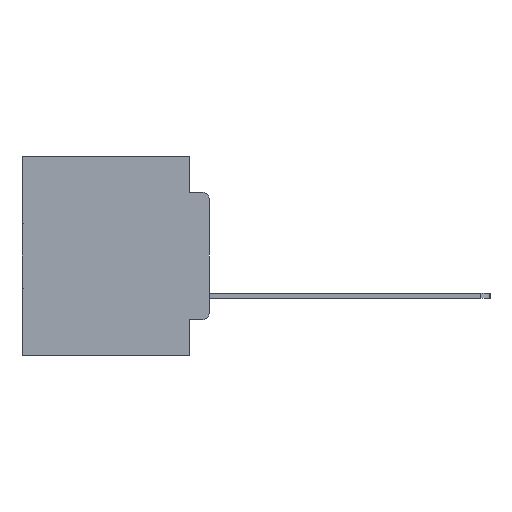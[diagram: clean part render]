
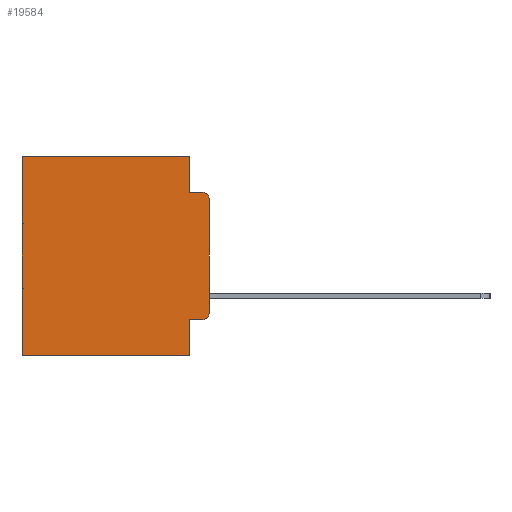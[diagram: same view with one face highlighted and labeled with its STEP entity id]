
A CAD part, left-side view. The second image highlights one B-rep face of the part: STEP entity #19584.
In plain terms, the highlighted planar face has unit normal (-1, 0, 0).
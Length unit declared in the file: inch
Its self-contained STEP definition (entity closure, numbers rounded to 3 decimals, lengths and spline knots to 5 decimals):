
#399 = CARTESIAN_POINT ( 'NONE',  ( 0.298, 0.473, -0.5 ) ) ;
#1230 = VERTEX_POINT ( 'NONE', #14262 ) ;
#1548 = CARTESIAN_POINT ( 'NONE',  ( 0.298, 0., -0.5 ) ) ;
#1728 = DIRECTION ( 'NONE',  ( 0., -1., 0. ) ) ;
#1893 = EDGE_CURVE ( 'NONE', #27802, #9238, #28339, .T. ) ;
#2396 = LINE ( 'NONE', #1548, #15229 ) ;
#2546 = CARTESIAN_POINT ( 'NONE',  ( 0.298, 0.02, -0.4115 ) ) ;
#2710 = CARTESIAN_POINT ( 'NONE',  ( 0.298, 0.051, -0.5 ) ) ;
#2961 = CARTESIAN_POINT ( 'NONE',  ( 0.298, 0.051, -0.0885 ) ) ;
#3117 = DIRECTION ( 'NONE',  ( 1., 0., 0. ) ) ;
#3260 = EDGE_LOOP ( 'NONE', ( #10660, #15494, #16611, #5345, #18315, #19833, #30527, #13112, #24665, #4795 ) ) ;
#3614 = DIRECTION ( 'NONE',  ( -1., 0., 0. ) ) ;
#4443 = CARTESIAN_POINT ( 'NONE',  ( 0.298, 0., 0. ) ) ;
#4523 = VERTEX_POINT ( 'NONE', #399 ) ;
#4795 = ORIENTED_EDGE ( 'NONE', *, *, #14055, .T. ) ;
#5158 = EDGE_CURVE ( 'NONE', #26946, #17206, #25175, .T. ) ;
#5345 = ORIENTED_EDGE ( 'NONE', *, *, #13250, .F. ) ;
#5708 = AXIS2_PLACEMENT_3D ( 'NONE', #12747, #29348, #15118 ) ;
#6300 = VERTEX_POINT ( 'NONE', #28837 ) ;
#6594 = VECTOR ( 'NONE', #21126, 39.37008 ) ;
#6880 = CARTESIAN_POINT ( 'NONE',  ( 0.298, 0.473, 0. ) ) ;
#7714 = DIRECTION ( 'NONE',  ( 0., 1., 0. ) ) ;
#8051 = VERTEX_POINT ( 'NONE', #2710 ) ;
#9105 = CARTESIAN_POINT ( 'NONE',  ( 0.298, 0.051, 0. ) ) ;
#9238 = VERTEX_POINT ( 'NONE', #14763 ) ;
#9301 = DIRECTION ( 'NONE',  ( 0., 0., -1. ) ) ;
#9405 = AXIS2_PLACEMENT_3D ( 'NONE', #18001, #3614, #20428 ) ;
#10660 = ORIENTED_EDGE ( 'NONE', *, *, #1893, .F. ) ;
#10932 = AXIS2_PLACEMENT_3D ( 'NONE', #17502, #3117, #19942 ) ;
#11236 = VECTOR ( 'NONE', #21817, 39.37008 ) ;
#12475 = CIRCLE ( 'NONE', #9405, 0.02 ) ;
#12482 = LINE ( 'NONE', #29075, #24395 ) ;
#12747 = CARTESIAN_POINT ( 'NONE',  ( 0.298, 0.02, -0.3915 ) ) ;
#13112 = ORIENTED_EDGE ( 'NONE', *, *, #17889, .F. ) ;
#13146 = EDGE_CURVE ( 'NONE', #8051, #4523, #2396, .T. ) ;
#13250 = EDGE_CURVE ( 'NONE', #25063, #26946, #18600, .T. ) ;
#13692 = CIRCLE ( 'NONE', #5708, 0.02 ) ;
#14055 = EDGE_CURVE ( 'NONE', #22486, #9238, #13692, .T. ) ;
#14067 = VECTOR ( 'NONE', #9301, 39.37008 ) ;
#14262 = CARTESIAN_POINT ( 'NONE',  ( 0.298, 0.473, 0. ) ) ;
#14763 = CARTESIAN_POINT ( 'NONE',  ( 0.298, 0., -0.3915 ) ) ;
#15104 = PLANE ( 'NONE',  #10932 ) ;
#15118 = DIRECTION ( 'NONE',  ( 0., 0., -1. ) ) ;
#15187 = VECTOR ( 'NONE', #1728, 39.37008 ) ;
#15229 = VECTOR ( 'NONE', #18423, 39.37008 ) ;
#15494 = ORIENTED_EDGE ( 'NONE', *, *, #28383, .T. ) ;
#15580 = EDGE_CURVE ( 'NONE', #25063, #1230, #12482, .T. ) ;
#15688 = VECTOR ( 'NONE', #21330, 39.37008 ) ;
#16611 = ORIENTED_EDGE ( 'NONE', *, *, #5158, .F. ) ;
#17206 = VERTEX_POINT ( 'NONE', #23819 ) ;
#17361 = DIRECTION ( 'NONE',  ( 0., -1., 0. ) ) ;
#17502 = CARTESIAN_POINT ( 'NONE',  ( 0.298, 0., 0. ) ) ;
#17818 = CARTESIAN_POINT ( 'NONE',  ( 0.298, 0., -0.1085 ) ) ;
#17889 = EDGE_CURVE ( 'NONE', #6300, #8051, #22432, .T. ) ;
#18001 = CARTESIAN_POINT ( 'NONE',  ( 0.298, 0.02, -0.1085 ) ) ;
#18114 = VECTOR ( 'NONE', #17361, 39.37008 ) ;
#18204 = LINE ( 'NONE', #25669, #15187 ) ;
#18315 = ORIENTED_EDGE ( 'NONE', *, *, #15580, .T. ) ;
#18423 = DIRECTION ( 'NONE',  ( 0., 1., 0. ) ) ;
#18600 = LINE ( 'NONE', #25910, #6594 ) ;
#19226 = CARTESIAN_POINT ( 'NONE',  ( 0.298, 0.051, 0. ) ) ;
#19584 = ADVANCED_FACE ( 'NONE', ( #26059 ), #15104, .F. ) ;
#19833 = ORIENTED_EDGE ( 'NONE', *, *, #20341, .T. ) ;
#19942 = DIRECTION ( 'NONE',  ( 0., 0., -1. ) ) ;
#20341 = EDGE_CURVE ( 'NONE', #1230, #4523, #22661, .T. ) ;
#20428 = DIRECTION ( 'NONE',  ( 0., 0., -1. ) ) ;
#21126 = DIRECTION ( 'NONE',  ( 0., 0., -1. ) ) ;
#21330 = DIRECTION ( 'NONE',  ( 0., 0., -1. ) ) ;
#21522 = CARTESIAN_POINT ( 'NONE',  ( 0.298, 0.051, -0.0885 ) ) ;
#21817 = DIRECTION ( 'NONE',  ( 0., 0., -1. ) ) ;
#22432 = LINE ( 'NONE', #19226, #11236 ) ;
#22486 = VERTEX_POINT ( 'NONE', #2546 ) ;
#22661 = LINE ( 'NONE', #6880, #14067 ) ;
#23819 = CARTESIAN_POINT ( 'NONE',  ( 0.298, 0.02, -0.0885 ) ) ;
#24395 = VECTOR ( 'NONE', #7714, 39.37008 ) ;
#24665 = ORIENTED_EDGE ( 'NONE', *, *, #25683, .T. ) ;
#25063 = VERTEX_POINT ( 'NONE', #9105 ) ;
#25175 = LINE ( 'NONE', #2961, #18114 ) ;
#25669 = CARTESIAN_POINT ( 'NONE',  ( 0.298, 0.051, -0.4115 ) ) ;
#25683 = EDGE_CURVE ( 'NONE', #6300, #22486, #18204, .T. ) ;
#25910 = CARTESIAN_POINT ( 'NONE',  ( 0.298, 0.051, 0. ) ) ;
#26059 = FACE_OUTER_BOUND ( 'NONE', #3260, .T. ) ;
#26946 = VERTEX_POINT ( 'NONE', #21522 ) ;
#27802 = VERTEX_POINT ( 'NONE', #17818 ) ;
#28339 = LINE ( 'NONE', #4443, #15688 ) ;
#28383 = EDGE_CURVE ( 'NONE', #27802, #17206, #12475, .T. ) ;
#28837 = CARTESIAN_POINT ( 'NONE',  ( 0.298, 0.051, -0.4115 ) ) ;
#29075 = CARTESIAN_POINT ( 'NONE',  ( 0.298, 0., 0. ) ) ;
#29348 = DIRECTION ( 'NONE',  ( -1., 0., 0. ) ) ;
#30527 = ORIENTED_EDGE ( 'NONE', *, *, #13146, .F. ) ;
